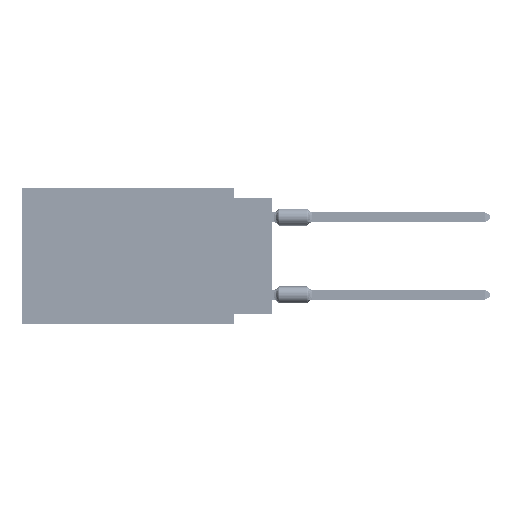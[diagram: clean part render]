
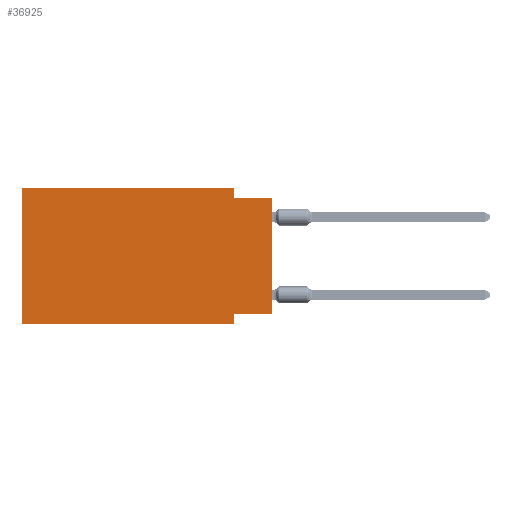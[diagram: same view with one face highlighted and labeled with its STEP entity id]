
A CAD part, left-side view. The second image highlights one B-rep face of the part: STEP entity #36925.
In plain terms, the highlighted planar face has unit normal (-1, 0, 0).
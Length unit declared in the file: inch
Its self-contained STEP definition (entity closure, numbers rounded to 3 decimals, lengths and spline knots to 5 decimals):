
#3247 = VERTEX_POINT ( 'NONE', #85759 ) ;
#3609 = VERTEX_POINT ( 'NONE', #63706 ) ;
#4071 = DIRECTION ( 'NONE',  ( 1., 0., 0. ) ) ;
#5474 = CARTESIAN_POINT ( 'NONE',  ( 0., 0., 0. ) ) ;
#5589 = EDGE_CURVE ( 'NONE', #3609, #80644, #66659, .T. ) ;
#6504 = ORIENTED_EDGE ( 'NONE', *, *, #64519, .F. ) ;
#6661 = VECTOR ( 'NONE', #42909, 39.37008 ) ;
#10287 = CARTESIAN_POINT ( 'NONE',  ( 0., 0.645, -0.35 ) ) ;
#10822 = CARTESIAN_POINT ( 'NONE',  ( 0., 0.645, 0. ) ) ;
#12667 = VERTEX_POINT ( 'NONE', #13299 ) ;
#13299 = CARTESIAN_POINT ( 'NONE',  ( 0., 0.645, 0. ) ) ;
#16713 = DIRECTION ( 'NONE',  ( 0., 0., -1. ) ) ;
#17061 = VECTOR ( 'NONE', #17279, 39.37008 ) ;
#17279 = DIRECTION ( 'NONE',  ( 0., -1., 0. ) ) ;
#18273 = DIRECTION ( 'NONE',  ( 0., 0., 1. ) ) ;
#18359 = VECTOR ( 'NONE', #65916, 39.37008 ) ;
#18457 = EDGE_CURVE ( 'NONE', #19089, #58424, #37084, .T. ) ;
#19089 = VERTEX_POINT ( 'NONE', #66395 ) ;
#19205 = LINE ( 'NONE', #10822, #50452 ) ;
#20588 = ORIENTED_EDGE ( 'NONE', *, *, #38382, .T. ) ;
#24151 = VERTEX_POINT ( 'NONE', #65164 ) ;
#24707 = ORIENTED_EDGE ( 'NONE', *, *, #25811, .F. ) ;
#25811 = EDGE_CURVE ( 'NONE', #24151, #3609, #72911, .T. ) ;
#27939 = AXIS2_PLACEMENT_3D ( 'NONE', #45673, #4071, #16713 ) ;
#27992 = CARTESIAN_POINT ( 'NONE',  ( 0., 0.1, 0. ) ) ;
#28898 = LINE ( 'NONE', #27992, #6661 ) ;
#31628 = CARTESIAN_POINT ( 'NONE',  ( 0., 0.645, 0. ) ) ;
#33768 = EDGE_LOOP ( 'NONE', ( #20588, #50045, #6504, #49853, #55831, #59888, #68962, #24707 ) ) ;
#36270 = EDGE_CURVE ( 'NONE', #57883, #12667, #19205, .T. ) ;
#36925 = ADVANCED_FACE ( 'NONE', ( #88200 ), #68103, .F. ) ;
#37084 = LINE ( 'NONE', #49709, #68535 ) ;
#38382 = EDGE_CURVE ( 'NONE', #24151, #58424, #40980, .T. ) ;
#40980 = LINE ( 'NONE', #5474, #66873 ) ;
#42909 = DIRECTION ( 'NONE',  ( 0., 0., -1. ) ) ;
#43969 = CARTESIAN_POINT ( 'NONE',  ( 0., 0., -0.325 ) ) ;
#44727 = LINE ( 'NONE', #31628, #61183 ) ;
#45542 = CARTESIAN_POINT ( 'NONE',  ( 0., 0.645, -0.35 ) ) ;
#45620 = DIRECTION ( 'NONE',  ( 0., 0., -1. ) ) ;
#45673 = CARTESIAN_POINT ( 'NONE',  ( 0., 0.645, 0. ) ) ;
#49709 = CARTESIAN_POINT ( 'NONE',  ( 0., 0., -0.025 ) ) ;
#49853 = ORIENTED_EDGE ( 'NONE', *, *, #57441, .F. ) ;
#50045 = ORIENTED_EDGE ( 'NONE', *, *, #18457, .F. ) ;
#50452 = VECTOR ( 'NONE', #18273, 39.37008 ) ;
#55521 = CARTESIAN_POINT ( 'NONE',  ( 0., 0.1, -0.35 ) ) ;
#55831 = ORIENTED_EDGE ( 'NONE', *, *, #36270, .F. ) ;
#57441 = EDGE_CURVE ( 'NONE', #12667, #3247, #44727, .T. ) ;
#57883 = VERTEX_POINT ( 'NONE', #45542 ) ;
#58424 = VERTEX_POINT ( 'NONE', #77963 ) ;
#59888 = ORIENTED_EDGE ( 'NONE', *, *, #64290, .T. ) ;
#60139 = DIRECTION ( 'NONE',  ( 0., -1., 0. ) ) ;
#61183 = VECTOR ( 'NONE', #60139, 39.37008 ) ;
#63706 = CARTESIAN_POINT ( 'NONE',  ( 0., 0.1, -0.325 ) ) ;
#64290 = EDGE_CURVE ( 'NONE', #57883, #80644, #81291, .T. ) ;
#64519 = EDGE_CURVE ( 'NONE', #3247, #19089, #28898, .T. ) ;
#65164 = CARTESIAN_POINT ( 'NONE',  ( 0., 0., -0.325 ) ) ;
#65916 = DIRECTION ( 'NONE',  ( 0., 1., 0. ) ) ;
#66395 = CARTESIAN_POINT ( 'NONE',  ( 0., 0.1, -0.025 ) ) ;
#66659 = LINE ( 'NONE', #81134, #74804 ) ;
#66873 = VECTOR ( 'NONE', #69490, 39.37008 ) ;
#68103 = PLANE ( 'NONE',  #27939 ) ;
#68535 = VECTOR ( 'NONE', #72134, 39.37008 ) ;
#68962 = ORIENTED_EDGE ( 'NONE', *, *, #5589, .F. ) ;
#69490 = DIRECTION ( 'NONE',  ( 0., 0., 1. ) ) ;
#72134 = DIRECTION ( 'NONE',  ( 0., -1., 0. ) ) ;
#72911 = LINE ( 'NONE', #43969, #18359 ) ;
#74804 = VECTOR ( 'NONE', #45620, 39.37008 ) ;
#77963 = CARTESIAN_POINT ( 'NONE',  ( 0., 0., -0.025 ) ) ;
#80644 = VERTEX_POINT ( 'NONE', #55521 ) ;
#81134 = CARTESIAN_POINT ( 'NONE',  ( 0., 0.1, -0.35 ) ) ;
#81291 = LINE ( 'NONE', #10287, #17061 ) ;
#85759 = CARTESIAN_POINT ( 'NONE',  ( 0., 0.1, 0. ) ) ;
#88200 = FACE_OUTER_BOUND ( 'NONE', #33768, .T. ) ;
